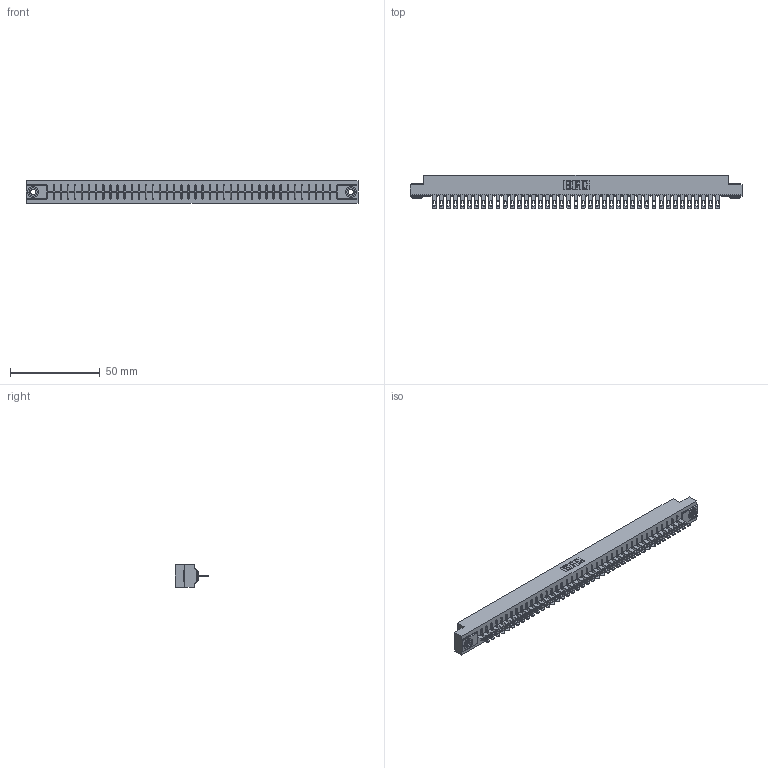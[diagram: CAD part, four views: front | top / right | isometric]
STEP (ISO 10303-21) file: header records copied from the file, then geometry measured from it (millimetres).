
FILE_DESCRIPTION (( 'STEP AP203' ), '1' );
FILE_NAME ('316-041-400-103.STEP', '2020-09-23T06:57:17', ( '' ), ( '' ), 'SwSTEP 2.0', 'SolidWorks 2020', '' );
FILE_SCHEMA (( 'CONFIG_CONTROL_DESIGN' ));
Length unit declared in the file: inch
Products named in the file (4): 306-290-001_100; 316-041-400-103; 345-250-002_345-250-002-102; 306 Part_.156 Dia
Assembly tree (44 placements, depth 2):
  316-041-400-103
    306 Part_.156 Dia
    306-290-001_100  x41
    345-250-002_345-250-002-102  x2
Bounding box: 185.47 x 18.87 x 12.7 mm (x, y, z)
Volume: 20643.1 mm3; surface area: 22141.7 mm2
Topology: 44 solids, 44 shells, 3284 faces, 9243 edges, 5938 vertices
Faces by surface type: plane 2142, cylinder 970, sphere 164, cone 8
Entity records: 39593 total; most frequent: CARTESIAN_POINT 6627, ORIENTED_EDGE 6562, DIRECTION 6549, EDGE_CURVE 3281, VECTOR 2557, LINE 2557, VERTEX_POINT 2074, AXIS2_PLACEMENT_3D 1996
